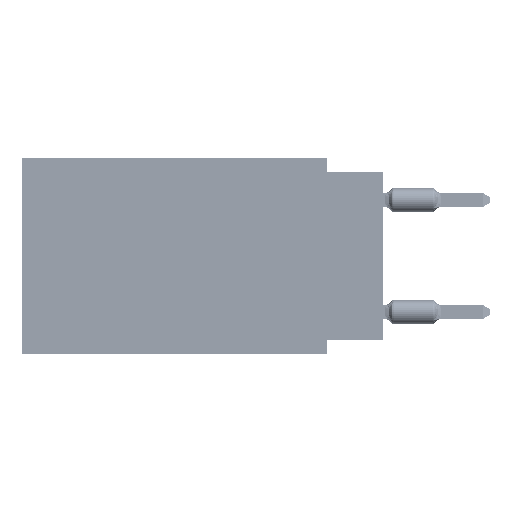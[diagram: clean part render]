
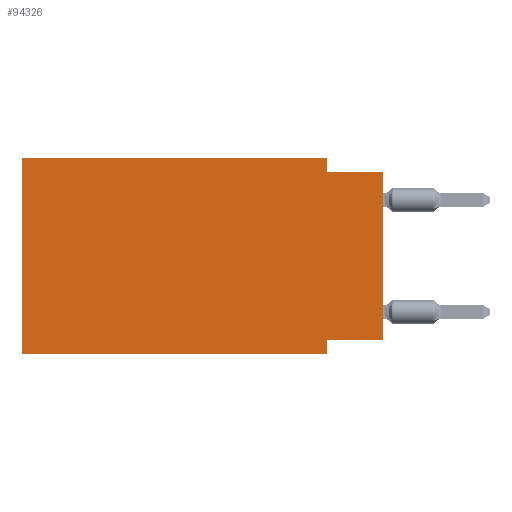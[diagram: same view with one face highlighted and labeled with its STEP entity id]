
A CAD part, left-side view. The second image highlights one B-rep face of the part: STEP entity #94326.
In plain terms, the highlighted planar face has unit normal (-1, 0, 0).
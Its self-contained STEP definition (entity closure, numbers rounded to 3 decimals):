
#1250 = ORIENTED_EDGE ( 'NONE', *, *, #66646, .F. ) ;
#2738 = VECTOR ( 'NONE', #12310, 1000. ) ;
#3003 = DIRECTION ( 'NONE',  ( 0., -1., 0. ) ) ;
#4480 = LINE ( 'NONE', #56862, #23859 ) ;
#7744 = LINE ( 'NONE', #67619, #27495 ) ;
#8658 = VECTOR ( 'NONE', #8826, 1000. ) ;
#8826 = DIRECTION ( 'NONE',  ( 0., 1., 0. ) ) ;
#10285 = ORIENTED_EDGE ( 'NONE', *, *, #83769, .T. ) ;
#12310 = DIRECTION ( 'NONE',  ( 0., -1., 0. ) ) ;
#13781 = CARTESIAN_POINT ( 'NONE',  ( 0., 2.54, -8.255 ) ) ;
#15340 = EDGE_CURVE ( 'NONE', #87668, #47554, #94854, .T. ) ;
#16314 = CARTESIAN_POINT ( 'NONE',  ( 0., 0., -8.255 ) ) ;
#17475 = CARTESIAN_POINT ( 'NONE',  ( 0., 16.383, 0. ) ) ;
#18695 = EDGE_CURVE ( 'NONE', #49228, #95372, #4480, .T. ) ;
#19351 = EDGE_LOOP ( 'NONE', ( #96172, #1250, #28104, #74260, #20211, #10285, #91370, #81731 ) ) ;
#20211 = ORIENTED_EDGE ( 'NONE', *, *, #70170, .F. ) ;
#20336 = PLANE ( 'NONE',  #24010 ) ;
#23859 = VECTOR ( 'NONE', #33450, 1000. ) ;
#24010 = AXIS2_PLACEMENT_3D ( 'NONE', #50750, #43276, #30772 ) ;
#24541 = VECTOR ( 'NONE', #3003, 1000. ) ;
#25584 = DIRECTION ( 'NONE',  ( 0., 0., 1. ) ) ;
#27495 = VECTOR ( 'NONE', #90533, 1000. ) ;
#28104 = ORIENTED_EDGE ( 'NONE', *, *, #18695, .F. ) ;
#29407 = LINE ( 'NONE', #83237, #30321 ) ;
#30275 = FACE_OUTER_BOUND ( 'NONE', #19351, .T. ) ;
#30321 = VECTOR ( 'NONE', #36418, 1000. ) ;
#30772 = DIRECTION ( 'NONE',  ( 0., 0., -1. ) ) ;
#33450 = DIRECTION ( 'NONE',  ( 0., 0., -1. ) ) ;
#36418 = DIRECTION ( 'NONE',  ( 0., 0., -1. ) ) ;
#39071 = CARTESIAN_POINT ( 'NONE',  ( 0., 16.383, 0. ) ) ;
#40800 = CARTESIAN_POINT ( 'NONE',  ( 0., 2.54, 0. ) ) ;
#41551 = CARTESIAN_POINT ( 'NONE',  ( 0., 0., 0. ) ) ;
#41861 = VECTOR ( 'NONE', #25584, 1000. ) ;
#42049 = DIRECTION ( 'NONE',  ( 0., 0., 1. ) ) ;
#43276 = DIRECTION ( 'NONE',  ( 1., 0., 0. ) ) ;
#44461 = CARTESIAN_POINT ( 'NONE',  ( 0., 16.383, -8.89 ) ) ;
#44947 = CARTESIAN_POINT ( 'NONE',  ( 0., 0., -8.255 ) ) ;
#45651 = VECTOR ( 'NONE', #42049, 1000. ) ;
#46545 = CARTESIAN_POINT ( 'NONE',  ( 0., 2.54, -8.89 ) ) ;
#47554 = VERTEX_POINT ( 'NONE', #54362 ) ;
#49228 = VERTEX_POINT ( 'NONE', #40800 ) ;
#50750 = CARTESIAN_POINT ( 'NONE',  ( 0., 16.383, 0. ) ) ;
#53192 = VERTEX_POINT ( 'NONE', #44461 ) ;
#54362 = CARTESIAN_POINT ( 'NONE',  ( 0., 0., -0.635 ) ) ;
#55337 = VERTEX_POINT ( 'NONE', #13781 ) ;
#56176 = VERTEX_POINT ( 'NONE', #65915 ) ;
#56862 = CARTESIAN_POINT ( 'NONE',  ( 0., 2.54, 0. ) ) ;
#61881 = LINE ( 'NONE', #17475, #24541 ) ;
#62800 = EDGE_CURVE ( 'NONE', #87668, #55337, #71148, .T. ) ;
#65915 = CARTESIAN_POINT ( 'NONE',  ( 0., 16.383, 0. ) ) ;
#66646 = EDGE_CURVE ( 'NONE', #95372, #47554, #74153, .T. ) ;
#67619 = CARTESIAN_POINT ( 'NONE',  ( 0., 16.383, -8.89 ) ) ;
#67987 = EDGE_CURVE ( 'NONE', #55337, #92303, #29407, .T. ) ;
#69402 = CARTESIAN_POINT ( 'NONE',  ( 0., 2.54, -0.635 ) ) ;
#70170 = EDGE_CURVE ( 'NONE', #53192, #56176, #84435, .T. ) ;
#71148 = LINE ( 'NONE', #16314, #8658 ) ;
#73427 = EDGE_CURVE ( 'NONE', #56176, #49228, #61881, .T. ) ;
#73658 = CARTESIAN_POINT ( 'NONE',  ( 0., 0., -0.635 ) ) ;
#74153 = LINE ( 'NONE', #73658, #2738 ) ;
#74260 = ORIENTED_EDGE ( 'NONE', *, *, #73427, .F. ) ;
#81731 = ORIENTED_EDGE ( 'NONE', *, *, #62800, .F. ) ;
#83237 = CARTESIAN_POINT ( 'NONE',  ( 0., 2.54, -8.89 ) ) ;
#83769 = EDGE_CURVE ( 'NONE', #53192, #92303, #7744, .T. ) ;
#84435 = LINE ( 'NONE', #39071, #41861 ) ;
#87668 = VERTEX_POINT ( 'NONE', #44947 ) ;
#90533 = DIRECTION ( 'NONE',  ( 0., -1., 0. ) ) ;
#91370 = ORIENTED_EDGE ( 'NONE', *, *, #67987, .F. ) ;
#92303 = VERTEX_POINT ( 'NONE', #46545 ) ;
#94326 = ADVANCED_FACE ( 'NONE', ( #30275 ), #20336, .F. ) ;
#94854 = LINE ( 'NONE', #41551, #45651 ) ;
#95372 = VERTEX_POINT ( 'NONE', #69402 ) ;
#96172 = ORIENTED_EDGE ( 'NONE', *, *, #15340, .T. ) ;
